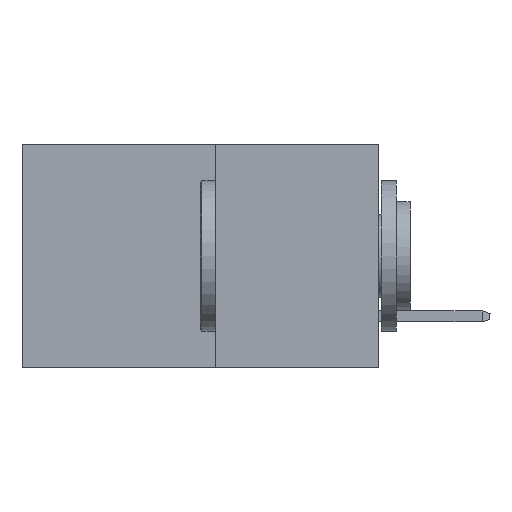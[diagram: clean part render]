
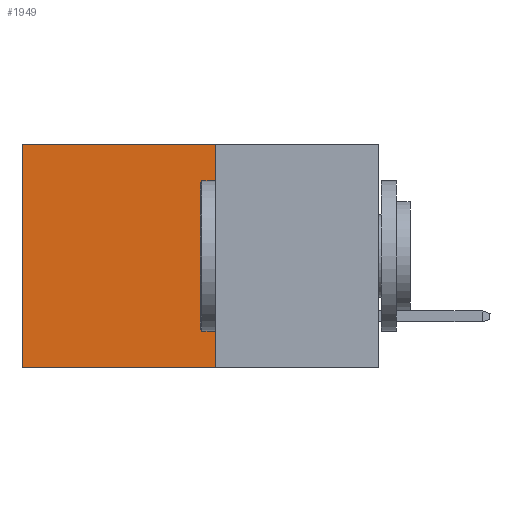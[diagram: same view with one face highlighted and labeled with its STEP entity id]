
A CAD part, left-side view. The second image highlights one B-rep face of the part: STEP entity #1949.
In plain terms, the highlighted planar face has unit normal (-1, 0, 0).
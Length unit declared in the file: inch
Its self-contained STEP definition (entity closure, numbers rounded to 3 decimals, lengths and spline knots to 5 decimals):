
#103 = VECTOR ( 'NONE', #4098, 39.37008 ) ;
#129 = EDGE_LOOP ( 'NONE', ( #4246, #11346, #5090, #16988 ) ) ;
#667 = CARTESIAN_POINT ( 'NONE',  ( 0.277, 0.59, -0.37 ) ) ;
#784 = LINE ( 'NONE', #667, #14503 ) ;
#1057 = LINE ( 'NONE', #3659, #14363 ) ;
#1623 = CARTESIAN_POINT ( 'NONE',  ( 0.277, 0.27, 0. ) ) ;
#1949 = ADVANCED_FACE ( 'NONE', ( #3866 ), #14717, .F. ) ;
#2604 = CARTESIAN_POINT ( 'NONE',  ( 0.277, 0.59, -0.37 ) ) ;
#2651 = CARTESIAN_POINT ( 'NONE',  ( 0.277, 0.27, -0.37 ) ) ;
#3659 = CARTESIAN_POINT ( 'NONE',  ( 0.277, 0.27, 0. ) ) ;
#3866 = FACE_OUTER_BOUND ( 'NONE', #129, .T. ) ;
#3999 = DIRECTION ( 'NONE',  ( 0., 0., -1. ) ) ;
#4098 = DIRECTION ( 'NONE',  ( 0., 1., 0. ) ) ;
#4179 = DIRECTION ( 'NONE',  ( 0., 1., 0. ) ) ;
#4246 = ORIENTED_EDGE ( 'NONE', *, *, #15972, .T. ) ;
#4273 = CARTESIAN_POINT ( 'NONE',  ( 0.277, 0.27, -0.37 ) ) ;
#4482 = VERTEX_POINT ( 'NONE', #1623 ) ;
#5090 = ORIENTED_EDGE ( 'NONE', *, *, #11548, .F. ) ;
#5121 = VERTEX_POINT ( 'NONE', #2604 ) ;
#5488 = CARTESIAN_POINT ( 'NONE',  ( 0.277, 0.59, 0. ) ) ;
#5657 = CARTESIAN_POINT ( 'NONE',  ( 0.277, 0.27, -0.37 ) ) ;
#7548 = DIRECTION ( 'NONE',  ( 0., 0., -1. ) ) ;
#8319 = VERTEX_POINT ( 'NONE', #5657 ) ;
#8377 = EDGE_CURVE ( 'NONE', #8319, #5121, #10823, .T. ) ;
#9110 = EDGE_CURVE ( 'NONE', #4482, #10214, #1057, .T. ) ;
#9411 = LINE ( 'NONE', #2651, #15863 ) ;
#9899 = AXIS2_PLACEMENT_3D ( 'NONE', #12254, #14806, #15219 ) ;
#10214 = VERTEX_POINT ( 'NONE', #5488 ) ;
#10823 = LINE ( 'NONE', #4273, #103 ) ;
#11346 = ORIENTED_EDGE ( 'NONE', *, *, #8377, .F. ) ;
#11548 = EDGE_CURVE ( 'NONE', #4482, #8319, #9411, .T. ) ;
#12254 = CARTESIAN_POINT ( 'NONE',  ( 0.277, 0.27, -0.37 ) ) ;
#14363 = VECTOR ( 'NONE', #4179, 39.37008 ) ;
#14503 = VECTOR ( 'NONE', #7548, 39.37008 ) ;
#14717 = PLANE ( 'NONE',  #9899 ) ;
#14806 = DIRECTION ( 'NONE',  ( 1., 0., 0. ) ) ;
#15219 = DIRECTION ( 'NONE',  ( 0., 0., -1. ) ) ;
#15863 = VECTOR ( 'NONE', #3999, 39.37008 ) ;
#15972 = EDGE_CURVE ( 'NONE', #10214, #5121, #784, .T. ) ;
#16988 = ORIENTED_EDGE ( 'NONE', *, *, #9110, .T. ) ;
